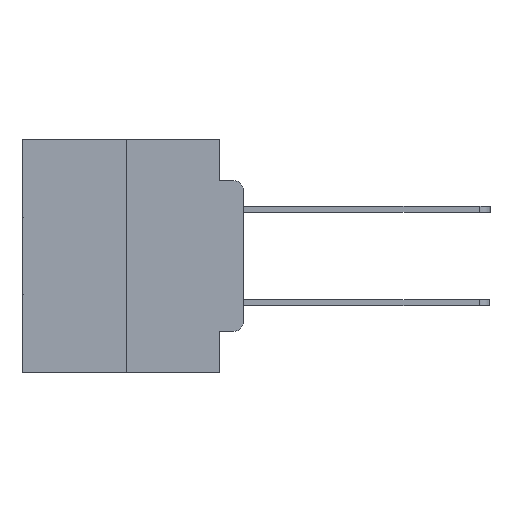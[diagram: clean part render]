
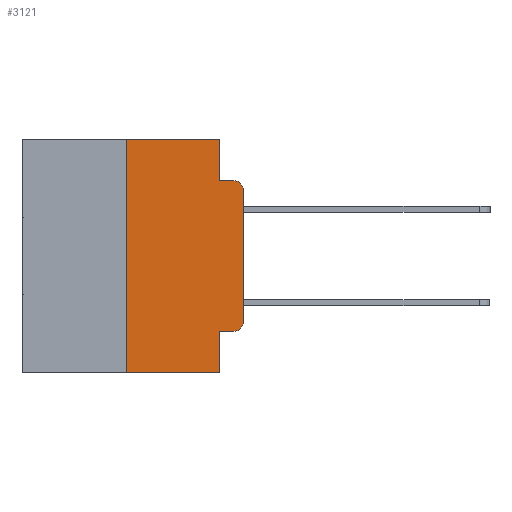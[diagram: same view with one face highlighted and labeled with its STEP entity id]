
A CAD part, left-side view. The second image highlights one B-rep face of the part: STEP entity #3121.
In plain terms, the highlighted planar face has unit normal (-1, 0, 0).
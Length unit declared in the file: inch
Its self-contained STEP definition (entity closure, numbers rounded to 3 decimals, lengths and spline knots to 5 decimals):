
#436 = LINE ( 'NONE', #29209, #12385 ) ;
#479 = LINE ( 'NONE', #15930, #6916 ) ;
#591 = VERTEX_POINT ( 'NONE', #23691 ) ;
#858 = DIRECTION ( 'NONE',  ( 0., -1., 0. ) ) ;
#964 = CARTESIAN_POINT ( 'NONE',  ( 0., 0.473, -0.5 ) ) ;
#1249 = VERTEX_POINT ( 'NONE', #19693 ) ;
#1396 = VERTEX_POINT ( 'NONE', #15610 ) ;
#1822 = AXIS2_PLACEMENT_3D ( 'NONE', #9567, #25900, #11929 ) ;
#1950 = CARTESIAN_POINT ( 'NONE',  ( 0., 0.051, -0.4115 ) ) ;
#3121 = ADVANCED_FACE ( 'NONE', ( #21749 ), #23988, .F. ) ;
#3783 = CARTESIAN_POINT ( 'NONE',  ( 0., 0.25, 0. ) ) ;
#4138 = VERTEX_POINT ( 'NONE', #20966 ) ;
#4141 = EDGE_CURVE ( 'NONE', #1249, #4708, #17957, .T. ) ;
#4518 = DIRECTION ( 'NONE',  ( -1., 0., 0. ) ) ;
#4708 = VERTEX_POINT ( 'NONE', #17366 ) ;
#4741 = LINE ( 'NONE', #1950, #10270 ) ;
#4953 = EDGE_CURVE ( 'NONE', #9130, #591, #479, .T. ) ;
#5135 = EDGE_CURVE ( 'NONE', #4708, #15791, #25919, .T. ) ;
#5147 = DIRECTION ( 'NONE',  ( 0., -1., 0. ) ) ;
#5412 = AXIS2_PLACEMENT_3D ( 'NONE', #16957, #26314, #12352 ) ;
#5441 = CARTESIAN_POINT ( 'NONE',  ( 0., 0.25, 0. ) ) ;
#5712 = CARTESIAN_POINT ( 'NONE',  ( 0., 0.051, -0.5 ) ) ;
#6916 = VECTOR ( 'NONE', #29819, 39.37008 ) ;
#7383 = CIRCLE ( 'NONE', #18036, 0.02 ) ;
#8546 = LINE ( 'NONE', #8893, #13999 ) ;
#8893 = CARTESIAN_POINT ( 'NONE',  ( 0., 0.051, 0. ) ) ;
#9130 = VERTEX_POINT ( 'NONE', #9676 ) ;
#9567 = CARTESIAN_POINT ( 'NONE',  ( 0., 0.02, -0.1085 ) ) ;
#9676 = CARTESIAN_POINT ( 'NONE',  ( 0., 0.051, 0. ) ) ;
#10270 = VECTOR ( 'NONE', #20787, 39.37008 ) ;
#10285 = EDGE_CURVE ( 'NONE', #591, #15791, #14661, .T. ) ;
#11249 = DIRECTION ( 'NONE',  ( 0., 0., -1. ) ) ;
#11280 = EDGE_CURVE ( 'NONE', #24822, #1396, #4741, .T. ) ;
#11748 = VECTOR ( 'NONE', #23313, 39.37008 ) ;
#11929 = DIRECTION ( 'NONE',  ( 0., 0., -1. ) ) ;
#12352 = DIRECTION ( 'NONE',  ( 0., 0., -1. ) ) ;
#12385 = VECTOR ( 'NONE', #17632, 39.37008 ) ;
#13012 = EDGE_CURVE ( 'NONE', #21705, #9130, #436, .T. ) ;
#13732 = VERTEX_POINT ( 'NONE', #5712 ) ;
#13739 = EDGE_CURVE ( 'NONE', #4138, #13732, #29074, .T. ) ;
#13901 = CARTESIAN_POINT ( 'NONE',  ( 0., 0., 0. ) ) ;
#13999 = VECTOR ( 'NONE', #11249, 39.37008 ) ;
#14661 = LINE ( 'NONE', #19209, #27084 ) ;
#15610 = CARTESIAN_POINT ( 'NONE',  ( 0., 0.02, -0.4115 ) ) ;
#15791 = VERTEX_POINT ( 'NONE', #27788 ) ;
#15930 = CARTESIAN_POINT ( 'NONE',  ( 0., 0.051, 0. ) ) ;
#16329 = ORIENTED_EDGE ( 'NONE', *, *, #4141, .T. ) ;
#16411 = ORIENTED_EDGE ( 'NONE', *, *, #5135, .T. ) ;
#16728 = VECTOR ( 'NONE', #858, 39.37008 ) ;
#16957 = CARTESIAN_POINT ( 'NONE',  ( 0., 0.473, 0. ) ) ;
#16989 = ORIENTED_EDGE ( 'NONE', *, *, #10285, .F. ) ;
#17188 = ORIENTED_EDGE ( 'NONE', *, *, #4953, .F. ) ;
#17218 = ORIENTED_EDGE ( 'NONE', *, *, #13012, .F. ) ;
#17366 = CARTESIAN_POINT ( 'NONE',  ( 0., 0., -0.1085 ) ) ;
#17632 = DIRECTION ( 'NONE',  ( 0., -1., 0. ) ) ;
#17668 = ORIENTED_EDGE ( 'NONE', *, *, #23044, .F. ) ;
#17682 = EDGE_LOOP ( 'NONE', ( #16329, #16411, #16989, #17188, #17218, #17668, #17847, #18368, #19226, #19398 ) ) ;
#17847 = ORIENTED_EDGE ( 'NONE', *, *, #13739, .T. ) ;
#17957 = LINE ( 'NONE', #13901, #11748 ) ;
#18036 = AXIS2_PLACEMENT_3D ( 'NONE', #18557, #4518, #20915 ) ;
#18368 = ORIENTED_EDGE ( 'NONE', *, *, #25558, .F. ) ;
#18557 = CARTESIAN_POINT ( 'NONE',  ( 0., 0.02, -0.3915 ) ) ;
#19209 = CARTESIAN_POINT ( 'NONE',  ( 0., 0.051, -0.0885 ) ) ;
#19226 = ORIENTED_EDGE ( 'NONE', *, *, #11280, .T. ) ;
#19398 = ORIENTED_EDGE ( 'NONE', *, *, #26291, .T. ) ;
#19693 = CARTESIAN_POINT ( 'NONE',  ( 0., 0., -0.3915 ) ) ;
#20743 = VECTOR ( 'NONE', #28835, 39.37008 ) ;
#20787 = DIRECTION ( 'NONE',  ( 0., -1., 0. ) ) ;
#20915 = DIRECTION ( 'NONE',  ( 0., 0., -1. ) ) ;
#20966 = CARTESIAN_POINT ( 'NONE',  ( 0., 0.25, -0.5 ) ) ;
#21705 = VERTEX_POINT ( 'NONE', #3783 ) ;
#21749 = FACE_OUTER_BOUND ( 'NONE', #17682, .T. ) ;
#23044 = EDGE_CURVE ( 'NONE', #4138, #21705, #26943, .T. ) ;
#23313 = DIRECTION ( 'NONE',  ( 0., 0., 1. ) ) ;
#23691 = CARTESIAN_POINT ( 'NONE',  ( 0., 0.051, -0.0885 ) ) ;
#23988 = PLANE ( 'NONE',  #5412 ) ;
#24822 = VERTEX_POINT ( 'NONE', #29498 ) ;
#25558 = EDGE_CURVE ( 'NONE', #24822, #13732, #8546, .T. ) ;
#25900 = DIRECTION ( 'NONE',  ( -1., 0., 0. ) ) ;
#25919 = CIRCLE ( 'NONE', #1822, 0.02 ) ;
#26291 = EDGE_CURVE ( 'NONE', #1396, #1249, #7383, .T. ) ;
#26314 = DIRECTION ( 'NONE',  ( 1., 0., 0. ) ) ;
#26943 = LINE ( 'NONE', #5441, #20743 ) ;
#27084 = VECTOR ( 'NONE', #5147, 39.37008 ) ;
#27788 = CARTESIAN_POINT ( 'NONE',  ( 0., 0.02, -0.0885 ) ) ;
#28835 = DIRECTION ( 'NONE',  ( 0., 0., 1. ) ) ;
#29074 = LINE ( 'NONE', #964, #16728 ) ;
#29209 = CARTESIAN_POINT ( 'NONE',  ( 0., 0.473, 0. ) ) ;
#29498 = CARTESIAN_POINT ( 'NONE',  ( 0., 0.051, -0.4115 ) ) ;
#29819 = DIRECTION ( 'NONE',  ( 0., 0., -1. ) ) ;
